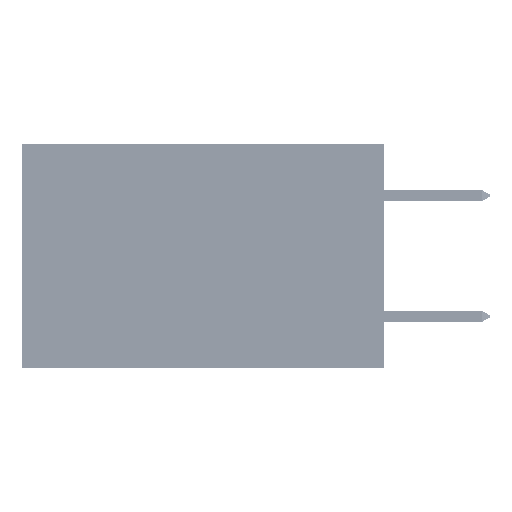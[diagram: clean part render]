
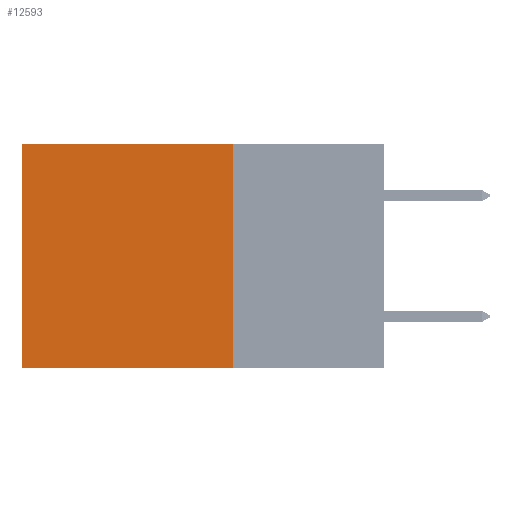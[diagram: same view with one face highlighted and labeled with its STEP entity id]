
A CAD part, left-side view. The second image highlights one B-rep face of the part: STEP entity #12593.
In plain terms, the highlighted planar face has unit normal (-1, 0, 0).
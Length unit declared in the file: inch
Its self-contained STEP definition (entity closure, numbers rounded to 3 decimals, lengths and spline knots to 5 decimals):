
#168 = CARTESIAN_POINT ( 'NONE',  ( 0.2875, 0.6, -0.37 ) ) ;
#3569 = EDGE_LOOP ( 'NONE', ( #32907, #10867, #25382, #26714 ) ) ;
#5403 = DIRECTION ( 'NONE',  ( 0., 1., 0. ) ) ;
#5696 = CARTESIAN_POINT ( 'NONE',  ( 0.2875, 0.25, 0. ) ) ;
#8016 = VECTOR ( 'NONE', #22064, 39.37008 ) ;
#10025 = PLANE ( 'NONE',  #37763 ) ;
#10867 = ORIENTED_EDGE ( 'NONE', *, *, #20234, .F. ) ;
#12593 = ADVANCED_FACE ( 'NONE', ( #37631 ), #10025, .F. ) ;
#13318 = VECTOR ( 'NONE', #16340, 39.37008 ) ;
#16033 = CARTESIAN_POINT ( 'NONE',  ( 0.2875, 0.25, 0. ) ) ;
#16340 = DIRECTION ( 'NONE',  ( 0., 0., -1. ) ) ;
#17138 = CARTESIAN_POINT ( 'NONE',  ( 0.2875, 0.25, 0. ) ) ;
#17237 = EDGE_CURVE ( 'NONE', #37696, #24308, #30531, .T. ) ;
#18206 = CARTESIAN_POINT ( 'NONE',  ( 0.2875, 0.6, 0. ) ) ;
#18497 = CARTESIAN_POINT ( 'NONE',  ( 0.2875, 0.25, -0.37 ) ) ;
#20234 = EDGE_CURVE ( 'NONE', #43129, #24308, #26682, .T. ) ;
#20710 = DIRECTION ( 'NONE',  ( 0., 0., -1. ) ) ;
#21998 = LINE ( 'NONE', #16033, #31183 ) ;
#22064 = DIRECTION ( 'NONE',  ( 0., 1., 0. ) ) ;
#23854 = CARTESIAN_POINT ( 'NONE',  ( 0.2875, 0.25, 0. ) ) ;
#24308 = VERTEX_POINT ( 'NONE', #168 ) ;
#25382 = ORIENTED_EDGE ( 'NONE', *, *, #44444, .F. ) ;
#26407 = CARTESIAN_POINT ( 'NONE',  ( 0.2875, 0.25, -0.37 ) ) ;
#26682 = LINE ( 'NONE', #18497, #8016 ) ;
#26714 = ORIENTED_EDGE ( 'NONE', *, *, #35256, .T. ) ;
#29456 = VECTOR ( 'NONE', #39156, 39.37008 ) ;
#30531 = LINE ( 'NONE', #18206, #29456 ) ;
#31183 = VECTOR ( 'NONE', #5403, 39.37008 ) ;
#32907 = ORIENTED_EDGE ( 'NONE', *, *, #17237, .T. ) ;
#33466 = CARTESIAN_POINT ( 'NONE',  ( 0.2875, 0.6, 0. ) ) ;
#35256 = EDGE_CURVE ( 'NONE', #40454, #37696, #21998, .T. ) ;
#37631 = FACE_OUTER_BOUND ( 'NONE', #3569, .T. ) ;
#37696 = VERTEX_POINT ( 'NONE', #33466 ) ;
#37763 = AXIS2_PLACEMENT_3D ( 'NONE', #17138, #41591, #20710 ) ;
#39156 = DIRECTION ( 'NONE',  ( 0., 0., -1. ) ) ;
#40180 = LINE ( 'NONE', #5696, #13318 ) ;
#40454 = VERTEX_POINT ( 'NONE', #23854 ) ;
#41591 = DIRECTION ( 'NONE',  ( 1., 0., 0. ) ) ;
#43129 = VERTEX_POINT ( 'NONE', #26407 ) ;
#44444 = EDGE_CURVE ( 'NONE', #40454, #43129, #40180, .T. ) ;
